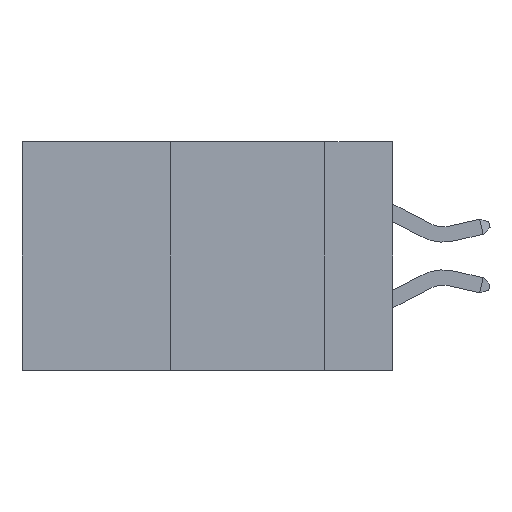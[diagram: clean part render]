
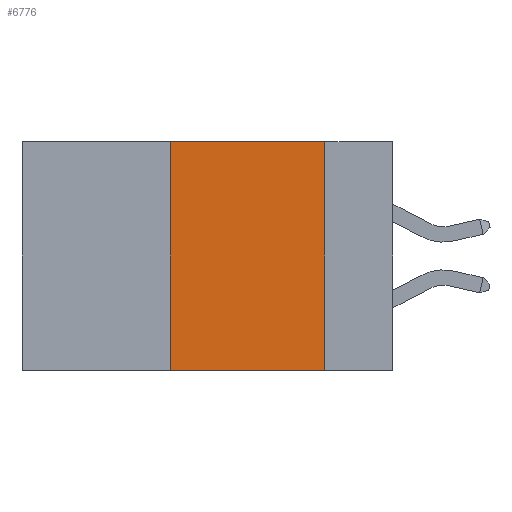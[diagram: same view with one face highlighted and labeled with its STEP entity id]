
A CAD part, left-side view. The second image highlights one B-rep face of the part: STEP entity #6776.
In plain terms, the highlighted planar face has unit normal (-1, 0, 0).
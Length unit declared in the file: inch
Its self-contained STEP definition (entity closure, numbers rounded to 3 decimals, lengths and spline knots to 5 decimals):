
#464 = ORIENTED_EDGE ( 'NONE', *, *, #1379, .F. ) ;
#977 = CARTESIAN_POINT ( 'NONE',  ( 0., 0.6, 0. ) ) ;
#1379 = EDGE_CURVE ( 'NONE', #8582, #10080, #16227, .T. ) ;
#1798 = CARTESIAN_POINT ( 'NONE',  ( 0., 0.11, 0. ) ) ;
#3291 = VECTOR ( 'NONE', #20875, 39.37008 ) ;
#3679 = CARTESIAN_POINT ( 'NONE',  ( 0., 0.11, 0. ) ) ;
#3731 = CARTESIAN_POINT ( 'NONE',  ( 0., 0.6, -0.37 ) ) ;
#3897 = CARTESIAN_POINT ( 'NONE',  ( 0., 0.11, -0.37 ) ) ;
#4998 = LINE ( 'NONE', #3731, #3291 ) ;
#5194 = ORIENTED_EDGE ( 'NONE', *, *, #9429, .T. ) ;
#5526 = LINE ( 'NONE', #19227, #9266 ) ;
#6052 = DIRECTION ( 'NONE',  ( 0., 0., -1. ) ) ;
#6370 = CARTESIAN_POINT ( 'NONE',  ( 0., 0.36, -0.37 ) ) ;
#6432 = CARTESIAN_POINT ( 'NONE',  ( 0., 0.6, 0. ) ) ;
#6545 = DIRECTION ( 'NONE',  ( 0., 0., -1. ) ) ;
#6776 = ADVANCED_FACE ( 'NONE', ( #11308 ), #9631, .F. ) ;
#8582 = VERTEX_POINT ( 'NONE', #26269 ) ;
#8887 = ORIENTED_EDGE ( 'NONE', *, *, #11914, .F. ) ;
#8935 = ORIENTED_EDGE ( 'NONE', *, *, #25790, .F. ) ;
#9266 = VECTOR ( 'NONE', #10733, 39.37008 ) ;
#9429 = EDGE_CURVE ( 'NONE', #15830, #26752, #4998, .T. ) ;
#9631 = PLANE ( 'NONE',  #14433 ) ;
#10080 = VERTEX_POINT ( 'NONE', #1798 ) ;
#10733 = DIRECTION ( 'NONE',  ( 0., 0., 1. ) ) ;
#11308 = FACE_OUTER_BOUND ( 'NONE', #25038, .T. ) ;
#11914 = EDGE_CURVE ( 'NONE', #10080, #26752, #23260, .T. ) ;
#14433 = AXIS2_PLACEMENT_3D ( 'NONE', #977, #19785, #6545 ) ;
#15830 = VERTEX_POINT ( 'NONE', #6370 ) ;
#16227 = LINE ( 'NONE', #6432, #25028 ) ;
#19227 = CARTESIAN_POINT ( 'NONE',  ( 0., 0.36, 0. ) ) ;
#19785 = DIRECTION ( 'NONE',  ( 1., 0., 0. ) ) ;
#20875 = DIRECTION ( 'NONE',  ( 0., -1., 0. ) ) ;
#21378 = DIRECTION ( 'NONE',  ( 0., -1., 0. ) ) ;
#23260 = LINE ( 'NONE', #3679, #27302 ) ;
#25028 = VECTOR ( 'NONE', #21378, 39.37008 ) ;
#25038 = EDGE_LOOP ( 'NONE', ( #8887, #464, #8935, #5194 ) ) ;
#25790 = EDGE_CURVE ( 'NONE', #15830, #8582, #5526, .T. ) ;
#26269 = CARTESIAN_POINT ( 'NONE',  ( 0., 0.36, 0. ) ) ;
#26752 = VERTEX_POINT ( 'NONE', #3897 ) ;
#27302 = VECTOR ( 'NONE', #6052, 39.37008 ) ;
